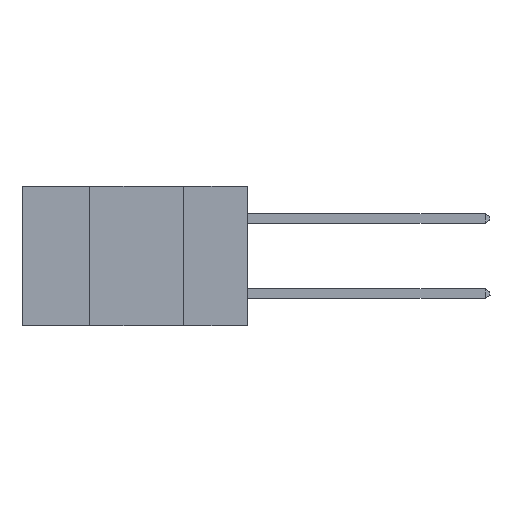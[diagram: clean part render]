
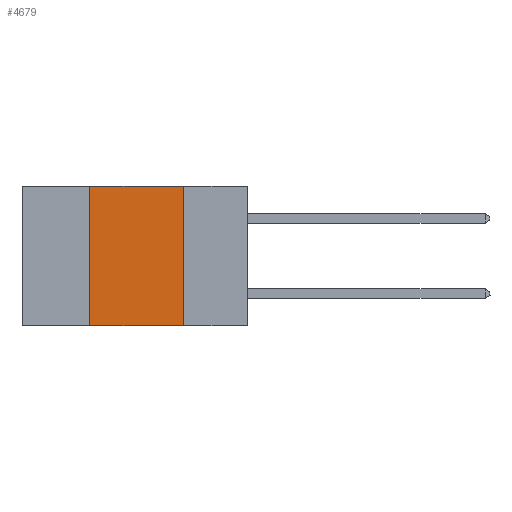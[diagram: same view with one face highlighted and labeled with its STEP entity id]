
A CAD part, left-side view. The second image highlights one B-rep face of the part: STEP entity #4679.
In plain terms, the highlighted planar face has unit normal (-1, 0, 0).
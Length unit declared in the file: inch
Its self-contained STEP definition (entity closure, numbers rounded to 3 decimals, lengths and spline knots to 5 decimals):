
#3903 = CARTESIAN_POINT ( 'NONE',  ( 0., 0.6, 0. ) ) ;
#4072 = FACE_OUTER_BOUND ( 'NONE', #15635, .T. ) ;
#4670 = VERTEX_POINT ( 'NONE', #13663 ) ;
#4679 = ADVANCED_FACE ( 'NONE', ( #4072 ), #9845, .F. ) ;
#5774 = DIRECTION ( 'NONE',  ( 1., 0., 0. ) ) ;
#5986 = CARTESIAN_POINT ( 'NONE',  ( 0., 0.17, -0.37 ) ) ;
#6383 = CARTESIAN_POINT ( 'NONE',  ( 0., 0.17, 0. ) ) ;
#6502 = ORIENTED_EDGE ( 'NONE', *, *, #20834, .F. ) ;
#6617 = VERTEX_POINT ( 'NONE', #5986 ) ;
#7873 = DIRECTION ( 'NONE',  ( 0., 0., -1. ) ) ;
#8553 = DIRECTION ( 'NONE',  ( 0., 0., 1. ) ) ;
#9829 = LINE ( 'NONE', #11677, #15422 ) ;
#9845 = PLANE ( 'NONE',  #11661 ) ;
#10567 = ORIENTED_EDGE ( 'NONE', *, *, #16651, .T. ) ;
#11650 = VERTEX_POINT ( 'NONE', #25171 ) ;
#11661 = AXIS2_PLACEMENT_3D ( 'NONE', #3903, #5774, #7873 ) ;
#11677 = CARTESIAN_POINT ( 'NONE',  ( 0., 0.6, 0. ) ) ;
#11793 = VECTOR ( 'NONE', #8553, 39.37008 ) ;
#13026 = DIRECTION ( 'NONE',  ( 0., -1., 0. ) ) ;
#13663 = CARTESIAN_POINT ( 'NONE',  ( 0., 0.42, -0.37 ) ) ;
#14145 = CARTESIAN_POINT ( 'NONE',  ( 0., 0.42, 0. ) ) ;
#14887 = VECTOR ( 'NONE', #20244, 39.37008 ) ;
#15422 = VECTOR ( 'NONE', #23925, 39.37008 ) ;
#15437 = EDGE_CURVE ( 'NONE', #4670, #18831, #17038, .T. ) ;
#15635 = EDGE_LOOP ( 'NONE', ( #16802, #6502, #18098, #10567 ) ) ;
#16651 = EDGE_CURVE ( 'NONE', #4670, #6617, #17270, .T. ) ;
#16802 = ORIENTED_EDGE ( 'NONE', *, *, #23912, .F. ) ;
#17038 = LINE ( 'NONE', #24344, #11793 ) ;
#17270 = LINE ( 'NONE', #22694, #21571 ) ;
#18098 = ORIENTED_EDGE ( 'NONE', *, *, #15437, .F. ) ;
#18831 = VERTEX_POINT ( 'NONE', #14145 ) ;
#20244 = DIRECTION ( 'NONE',  ( 0., 0., -1. ) ) ;
#20834 = EDGE_CURVE ( 'NONE', #18831, #11650, #9829, .T. ) ;
#21571 = VECTOR ( 'NONE', #13026, 39.37008 ) ;
#22694 = CARTESIAN_POINT ( 'NONE',  ( 0., 0.6, -0.37 ) ) ;
#23490 = LINE ( 'NONE', #6383, #14887 ) ;
#23912 = EDGE_CURVE ( 'NONE', #11650, #6617, #23490, .T. ) ;
#23925 = DIRECTION ( 'NONE',  ( 0., -1., 0. ) ) ;
#24344 = CARTESIAN_POINT ( 'NONE',  ( 0., 0.42, 0. ) ) ;
#25171 = CARTESIAN_POINT ( 'NONE',  ( 0., 0.17, 0. ) ) ;
